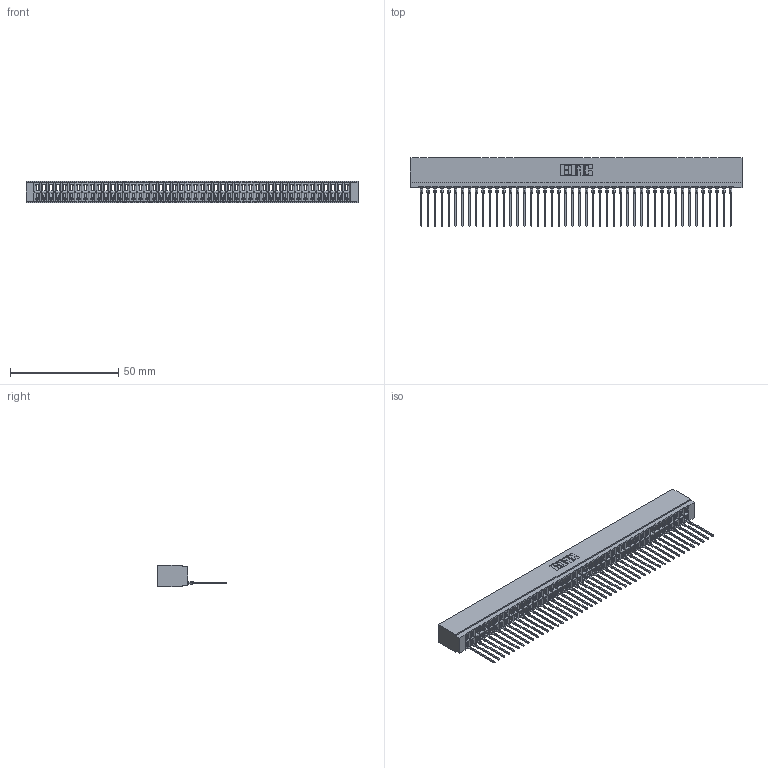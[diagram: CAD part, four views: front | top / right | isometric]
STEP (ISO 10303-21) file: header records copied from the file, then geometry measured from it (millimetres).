
FILE_DESCRIPTION (( 'STEP AP203' ), '1' );
FILE_NAME ('726-046-553-101.STEP', '2020-05-28T07:47:32', ( '' ), ( '' ), 'SwSTEP 2.0', 'SolidWorks 2020', '' );
FILE_SCHEMA (( 'CONFIG_CONTROL_DESIGN' ));
Length unit declared in the file: inch
Products named in the file (3): 726-046-553-101; 746-292-001_553; 726 Part_.515 Slot Depth - 01
Assembly tree (47 placements, depth 2):
  726-046-553-101
    726 Part_.515 Slot Depth - 01
    746-292-001_553  x46
Bounding box: 153.29 x 31.79 x 9.91 mm (x, y, z)
Volume: 13840.7 mm3; surface area: 22025.7 mm2
Topology: 47 solids, 47 shells, 5065 faces, 14385 edges, 9237 vertices
Faces by surface type: plane 2953, bspline 920, cylinder 916, torus 276
Entity records: 68951 total; most frequent: CARTESIAN_POINT 13919, ORIENTED_EDGE 12120, DIRECTION 10020, EDGE_CURVE 6060, VECTOR 5416, LINE 5416, VERTEX_POINT 4017, AXIS2_PLACEMENT_3D 2302
